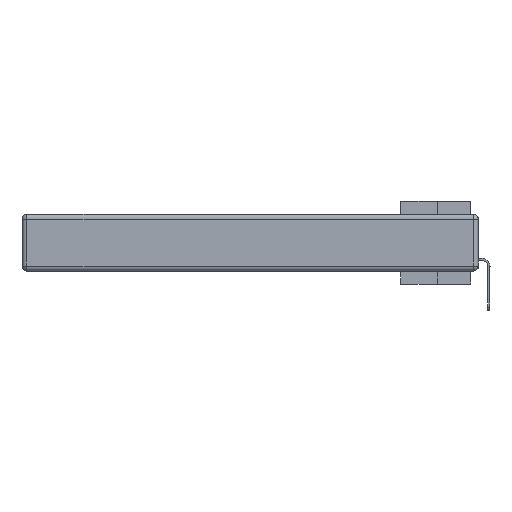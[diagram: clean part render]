
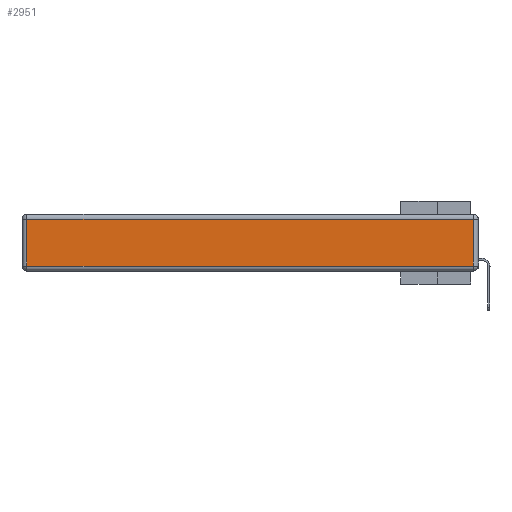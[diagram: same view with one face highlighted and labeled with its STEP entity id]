
A CAD part, left-side view. The second image highlights one B-rep face of the part: STEP entity #2951.
In plain terms, the highlighted planar face has unit normal (-1, 0, 0).
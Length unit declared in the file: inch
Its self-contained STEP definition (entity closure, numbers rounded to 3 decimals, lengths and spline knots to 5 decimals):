
#137 = EDGE_CURVE ( 'NONE', #26243, #22329, #4529, .T. ) ;
#936 = EDGE_CURVE ( 'NONE', #22329, #5712, #27882, .T. ) ;
#1373 = PLANE ( 'NONE',  #22157 ) ;
#1445 = EDGE_LOOP ( 'NONE', ( #18572, #6972, #3873, #17183 ) ) ;
#2951 = ADVANCED_FACE ( 'NONE', ( #15566 ), #1373, .T. ) ;
#3503 = LINE ( 'NONE', #8111, #16748 ) ;
#3772 = CARTESIAN_POINT ( 'NONE',  ( 0., 2.72, -0.313 ) ) ;
#3873 = ORIENTED_EDGE ( 'NONE', *, *, #29229, .T. ) ;
#4529 = LINE ( 'NONE', #27517, #25081 ) ;
#5712 = VERTEX_POINT ( 'NONE', #13294 ) ;
#6972 = ORIENTED_EDGE ( 'NONE', *, *, #14915, .T. ) ;
#8110 = DIRECTION ( 'NONE',  ( 0., 0., 1. ) ) ;
#8111 = CARTESIAN_POINT ( 'NONE',  ( 0., 0.03, -0.343 ) ) ;
#8682 = CARTESIAN_POINT ( 'NONE',  ( 0., 0.03, -0.03 ) ) ;
#9180 = CARTESIAN_POINT ( 'NONE',  ( 0., 2.72, -0.03 ) ) ;
#10392 = DIRECTION ( 'NONE',  ( 0., 1., 0. ) ) ;
#12986 = LINE ( 'NONE', #14811, #22158 ) ;
#13294 = CARTESIAN_POINT ( 'NONE',  ( 0., 0.03, -0.313 ) ) ;
#13722 = DIRECTION ( 'NONE',  ( 0., 0., -1. ) ) ;
#14811 = CARTESIAN_POINT ( 'NONE',  ( 0., 2.75, -0.03 ) ) ;
#14915 = EDGE_CURVE ( 'NONE', #5712, #22393, #3503, .T. ) ;
#15241 = VECTOR ( 'NONE', #30025, 39.37008 ) ;
#15566 = FACE_OUTER_BOUND ( 'NONE', #1445, .T. ) ;
#16748 = VECTOR ( 'NONE', #29217, 39.37008 ) ;
#17183 = ORIENTED_EDGE ( 'NONE', *, *, #137, .T. ) ;
#18572 = ORIENTED_EDGE ( 'NONE', *, *, #936, .T. ) ;
#20750 = CARTESIAN_POINT ( 'NONE',  ( 0., 0., -0.313 ) ) ;
#22157 = AXIS2_PLACEMENT_3D ( 'NONE', #24199, #24784, #8110 ) ;
#22158 = VECTOR ( 'NONE', #10392, 39.37008 ) ;
#22329 = VERTEX_POINT ( 'NONE', #3772 ) ;
#22393 = VERTEX_POINT ( 'NONE', #8682 ) ;
#24199 = CARTESIAN_POINT ( 'NONE',  ( 0., 0., -0.343 ) ) ;
#24784 = DIRECTION ( 'NONE',  ( -1., 0., 0. ) ) ;
#25081 = VECTOR ( 'NONE', #13722, 39.37008 ) ;
#26243 = VERTEX_POINT ( 'NONE', #9180 ) ;
#27517 = CARTESIAN_POINT ( 'NONE',  ( 0., 2.72, -0.343 ) ) ;
#27882 = LINE ( 'NONE', #20750, #15241 ) ;
#29217 = DIRECTION ( 'NONE',  ( 0., 0., 1. ) ) ;
#29229 = EDGE_CURVE ( 'NONE', #22393, #26243, #12986, .T. ) ;
#30025 = DIRECTION ( 'NONE',  ( 0., -1., 0. ) ) ;
